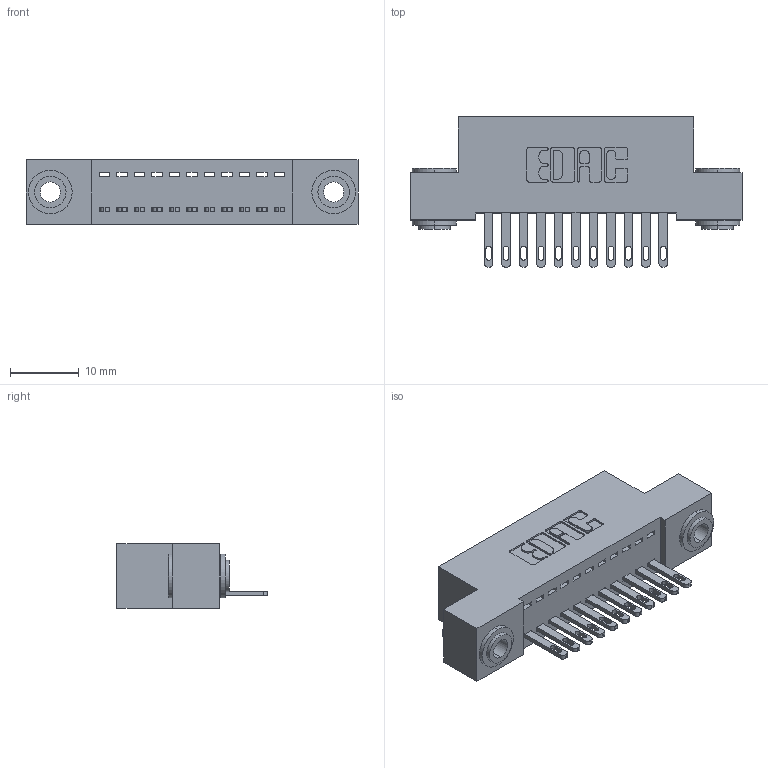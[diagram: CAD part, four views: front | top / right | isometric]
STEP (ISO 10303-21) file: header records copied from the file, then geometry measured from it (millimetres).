
FILE_DESCRIPTION (( 'STEP AP203' ), '1' );
FILE_NAME ('892-011-500-103.STEP', '2020-09-21T12:54:52', ( '' ), ( '' ), 'SwSTEP 2.0', 'SolidWorks 2020', '' );
FILE_SCHEMA (( 'CONFIG_CONTROL_DESIGN' ));
Length unit declared in the file: inch
Products named in the file (4): 892-011-500-103; 842 Part_.156 TH; 342-250-002_345-250-002-102; 345-292-001_345-293-100
Assembly tree (14 placements, depth 2):
  892-011-500-103
    842 Part_.156 TH
    345-292-001_345-293-100  x11
    342-250-002_345-250-002-102  x2
Bounding box: 48.26 x 21.85 x 9.4 mm (x, y, z)
Volume: 4146.9 mm3; surface area: 5758.5 mm2
Topology: 14 solids, 14 shells, 742 faces, 2223 edges, 1478 vertices
Faces by surface type: plane 472, cylinder 262, cone 8
Entity records: 11182 total; most frequent: CARTESIAN_POINT 1910, ORIENTED_EDGE 1850, DIRECTION 1709, EDGE_CURVE 925, VECTOR 769, LINE 769, VERTEX_POINT 614, AXIS2_PLACEMENT_3D 470
